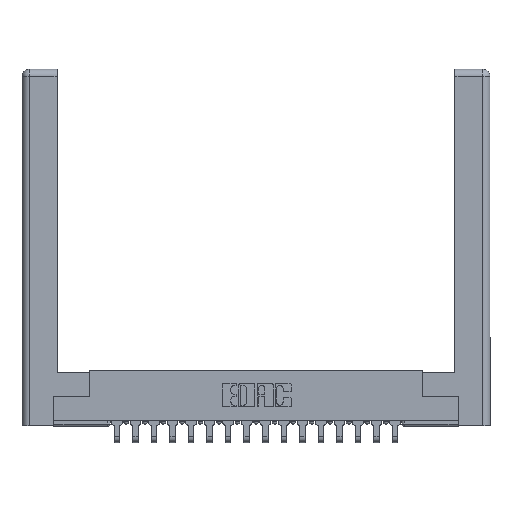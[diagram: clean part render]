
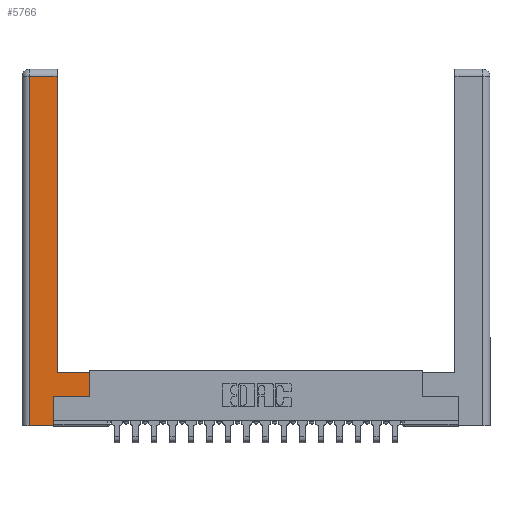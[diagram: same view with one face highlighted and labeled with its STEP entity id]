
A CAD part, top view. The second image highlights one B-rep face of the part: STEP entity #5766.
In plain terms, the highlighted planar face has unit normal (0, 0, 1).
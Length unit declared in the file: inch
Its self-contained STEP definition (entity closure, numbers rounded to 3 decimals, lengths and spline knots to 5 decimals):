
#153 = CARTESIAN_POINT ( 'NONE',  ( 0.0615, 2.94, 0. ) ) ;
#525 = CARTESIAN_POINT ( 'NONE',  ( 0., 0., 0. ) ) ;
#579 = LINE ( 'NONE', #8485, #19110 ) ;
#667 = CARTESIAN_POINT ( 'NONE',  ( 0.295, 0.45, 0. ) ) ;
#1018 = EDGE_CURVE ( 'NONE', #16109, #17333, #10566, .T. ) ;
#1059 = VERTEX_POINT ( 'NONE', #8546 ) ;
#2024 = LINE ( 'NONE', #4955, #12225 ) ;
#2047 = DIRECTION ( 'NONE',  ( 0., 0., -1. ) ) ;
#2398 = CARTESIAN_POINT ( 'NONE',  ( 0.265, 0.245, 0. ) ) ;
#2562 = DIRECTION ( 'NONE',  ( 0., 1., 0. ) ) ;
#3348 = ORIENTED_EDGE ( 'NONE', *, *, #6718, .T. ) ;
#3626 = CARTESIAN_POINT ( 'NONE',  ( 0.265, 0., 0. ) ) ;
#4143 = VECTOR ( 'NONE', #17252, 39.37008 ) ;
#4302 = EDGE_CURVE ( 'NONE', #5795, #16109, #2024, .T. ) ;
#4437 = VECTOR ( 'NONE', #16185, 39.37008 ) ;
#4538 = VECTOR ( 'NONE', #9602, 39.37008 ) ;
#4778 = CARTESIAN_POINT ( 'NONE',  ( 0.0615, 0., 0. ) ) ;
#4809 = ORIENTED_EDGE ( 'NONE', *, *, #1018, .T. ) ;
#4955 = CARTESIAN_POINT ( 'NONE',  ( 0.265, 0.245, 0. ) ) ;
#5156 = CARTESIAN_POINT ( 'NONE',  ( 0.565, 0.245, 0. ) ) ;
#5541 = VECTOR ( 'NONE', #18303, 39.37008 ) ;
#5766 = ADVANCED_FACE ( 'NONE', ( #15505 ), #9617, .F. ) ;
#5795 = VERTEX_POINT ( 'NONE', #3626 ) ;
#6021 = DIRECTION ( 'NONE',  ( -1., 0., 0. ) ) ;
#6462 = ORIENTED_EDGE ( 'NONE', *, *, #8493, .T. ) ;
#6718 = EDGE_CURVE ( 'NONE', #17333, #13576, #15010, .T. ) ;
#7499 = CARTESIAN_POINT ( 'NONE',  ( 0.295, 0.45, 0. ) ) ;
#8023 = DIRECTION ( 'NONE',  ( -1., 0., 0. ) ) ;
#8485 = CARTESIAN_POINT ( 'NONE',  ( 0.295, 3., 0. ) ) ;
#8489 = CARTESIAN_POINT ( 'NONE',  ( 0.265, 0., 0. ) ) ;
#8493 = EDGE_CURVE ( 'NONE', #18326, #5795, #10600, .T. ) ;
#8546 = CARTESIAN_POINT ( 'NONE',  ( 0.0615, 2.94, 0. ) ) ;
#8635 = LINE ( 'NONE', #7499, #5541 ) ;
#8779 = ORIENTED_EDGE ( 'NONE', *, *, #4302, .T. ) ;
#8799 = AXIS2_PLACEMENT_3D ( 'NONE', #525, #2047, #8023 ) ;
#9602 = DIRECTION ( 'NONE',  ( 0., 1., 0. ) ) ;
#9617 = PLANE ( 'NONE',  #8799 ) ;
#10566 = LINE ( 'NONE', #5156, #4143 ) ;
#10571 = VECTOR ( 'NONE', #18597, 39.37008 ) ;
#10600 = LINE ( 'NONE', #8489, #4437 ) ;
#11858 = EDGE_CURVE ( 'NONE', #13557, #1059, #15925, .T. ) ;
#12225 = VECTOR ( 'NONE', #12482, 39.37008 ) ;
#12355 = EDGE_LOOP ( 'NONE', ( #14410, #16572, #12859, #6462, #8779, #4809, #3348, #14388 ) ) ;
#12482 = DIRECTION ( 'NONE',  ( 0., 1., 0. ) ) ;
#12859 = ORIENTED_EDGE ( 'NONE', *, *, #18975, .T. ) ;
#13557 = VERTEX_POINT ( 'NONE', #14140 ) ;
#13576 = VERTEX_POINT ( 'NONE', #17201 ) ;
#14140 = CARTESIAN_POINT ( 'NONE',  ( 0.295, 2.94, 0. ) ) ;
#14244 = CARTESIAN_POINT ( 'NONE',  ( 0.565, 0.245, 0. ) ) ;
#14358 = EDGE_CURVE ( 'NONE', #19177, #13557, #579, .T. ) ;
#14388 = ORIENTED_EDGE ( 'NONE', *, *, #14601, .T. ) ;
#14410 = ORIENTED_EDGE ( 'NONE', *, *, #14358, .T. ) ;
#14601 = EDGE_CURVE ( 'NONE', #13576, #19177, #8635, .T. ) ;
#15010 = LINE ( 'NONE', #15620, #4538 ) ;
#15505 = FACE_OUTER_BOUND ( 'NONE', #12355, .T. ) ;
#15620 = CARTESIAN_POINT ( 'NONE',  ( 0.565, 0.45, 0. ) ) ;
#15925 = LINE ( 'NONE', #153, #19025 ) ;
#16109 = VERTEX_POINT ( 'NONE', #2398 ) ;
#16185 = DIRECTION ( 'NONE',  ( 1., 0., 0. ) ) ;
#16572 = ORIENTED_EDGE ( 'NONE', *, *, #11858, .T. ) ;
#17201 = CARTESIAN_POINT ( 'NONE',  ( 0.565, 0.45, 0. ) ) ;
#17252 = DIRECTION ( 'NONE',  ( 1., 0., 0. ) ) ;
#17333 = VERTEX_POINT ( 'NONE', #14244 ) ;
#18303 = DIRECTION ( 'NONE',  ( -1., 0., 0. ) ) ;
#18326 = VERTEX_POINT ( 'NONE', #4778 ) ;
#18528 = CARTESIAN_POINT ( 'NONE',  ( 0.0615, 0., 0. ) ) ;
#18597 = DIRECTION ( 'NONE',  ( 0., -1., 0. ) ) ;
#18668 = LINE ( 'NONE', #18528, #10571 ) ;
#18975 = EDGE_CURVE ( 'NONE', #1059, #18326, #18668, .T. ) ;
#19025 = VECTOR ( 'NONE', #6021, 39.37008 ) ;
#19110 = VECTOR ( 'NONE', #2562, 39.37008 ) ;
#19177 = VERTEX_POINT ( 'NONE', #667 ) ;
